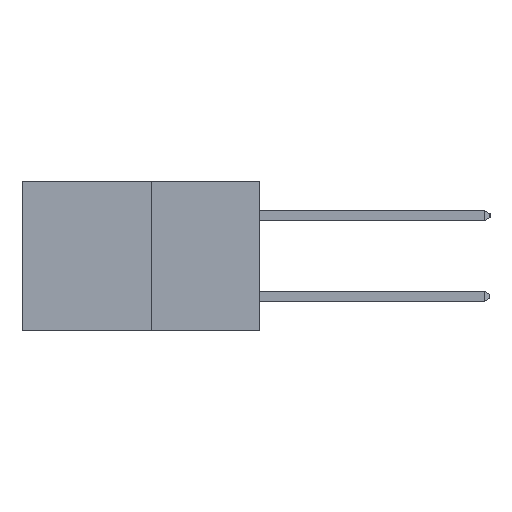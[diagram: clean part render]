
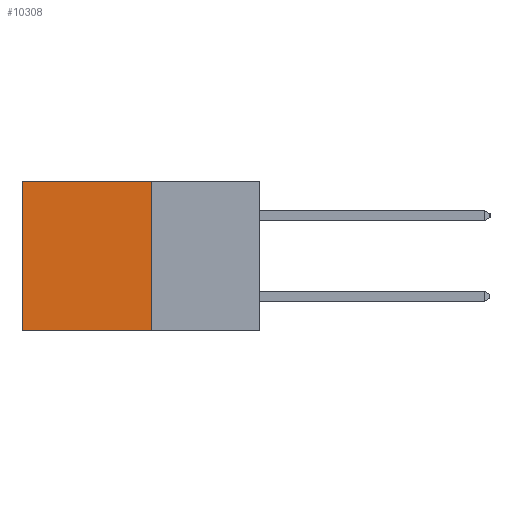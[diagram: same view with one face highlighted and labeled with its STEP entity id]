
A CAD part, left-side view. The second image highlights one B-rep face of the part: STEP entity #10308.
In plain terms, the highlighted planar face has unit normal (-1, 0, 0).
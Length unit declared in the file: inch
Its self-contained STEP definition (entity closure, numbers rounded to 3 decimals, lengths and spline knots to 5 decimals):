
#768 = EDGE_CURVE ( 'NONE', #7690, #11647, #1055, .T. ) ;
#964 = AXIS2_PLACEMENT_3D ( 'NONE', #8460, #11960, #5100 ) ;
#1055 = LINE ( 'NONE', #7065, #12526 ) ;
#1257 = EDGE_CURVE ( 'NONE', #11647, #1409, #9119, .T. ) ;
#1409 = VERTEX_POINT ( 'NONE', #1433 ) ;
#1433 = CARTESIAN_POINT ( 'NONE',  ( 0.277, 0.59, -0.37 ) ) ;
#1660 = PLANE ( 'NONE',  #964 ) ;
#1794 = VECTOR ( 'NONE', #13767, 39.37008 ) ;
#2709 = EDGE_CURVE ( 'NONE', #11717, #1409, #9311, .T. ) ;
#2859 = EDGE_CURVE ( 'NONE', #7690, #11717, #10181, .T. ) ;
#2971 = ORIENTED_EDGE ( 'NONE', *, *, #1257, .F. ) ;
#3276 = ORIENTED_EDGE ( 'NONE', *, *, #768, .F. ) ;
#3856 = ORIENTED_EDGE ( 'NONE', *, *, #2859, .T. ) ;
#4157 = ORIENTED_EDGE ( 'NONE', *, *, #2709, .T. ) ;
#4457 = VECTOR ( 'NONE', #10719, 39.37008 ) ;
#5100 = DIRECTION ( 'NONE',  ( 0., 0., -1. ) ) ;
#5514 = CARTESIAN_POINT ( 'NONE',  ( 0.277, 0.27, -0.37 ) ) ;
#6267 = VECTOR ( 'NONE', #10036, 39.37008 ) ;
#7065 = CARTESIAN_POINT ( 'NONE',  ( 0.277, 0.27, -0.37 ) ) ;
#7690 = VERTEX_POINT ( 'NONE', #10747 ) ;
#7897 = EDGE_LOOP ( 'NONE', ( #4157, #2971, #3276, #3856 ) ) ;
#8460 = CARTESIAN_POINT ( 'NONE',  ( 0.277, 0.27, -0.37 ) ) ;
#9119 = LINE ( 'NONE', #12412, #1794 ) ;
#9158 = CARTESIAN_POINT ( 'NONE',  ( 0.277, 0.59, -0.37 ) ) ;
#9311 = LINE ( 'NONE', #9158, #6267 ) ;
#10036 = DIRECTION ( 'NONE',  ( 0., 0., -1. ) ) ;
#10181 = LINE ( 'NONE', #10649, #4457 ) ;
#10308 = ADVANCED_FACE ( 'NONE', ( #10508 ), #1660, .F. ) ;
#10508 = FACE_OUTER_BOUND ( 'NONE', #7897, .T. ) ;
#10649 = CARTESIAN_POINT ( 'NONE',  ( 0.277, 0.27, 0. ) ) ;
#10719 = DIRECTION ( 'NONE',  ( 0., 1., 0. ) ) ;
#10747 = CARTESIAN_POINT ( 'NONE',  ( 0.277, 0.27, 0. ) ) ;
#10849 = DIRECTION ( 'NONE',  ( 0., 0., -1. ) ) ;
#11348 = CARTESIAN_POINT ( 'NONE',  ( 0.277, 0.59, 0. ) ) ;
#11647 = VERTEX_POINT ( 'NONE', #5514 ) ;
#11717 = VERTEX_POINT ( 'NONE', #11348 ) ;
#11960 = DIRECTION ( 'NONE',  ( 1., 0., 0. ) ) ;
#12412 = CARTESIAN_POINT ( 'NONE',  ( 0.277, 0.27, -0.37 ) ) ;
#12526 = VECTOR ( 'NONE', #10849, 39.37008 ) ;
#13767 = DIRECTION ( 'NONE',  ( 0., 1., 0. ) ) ;
